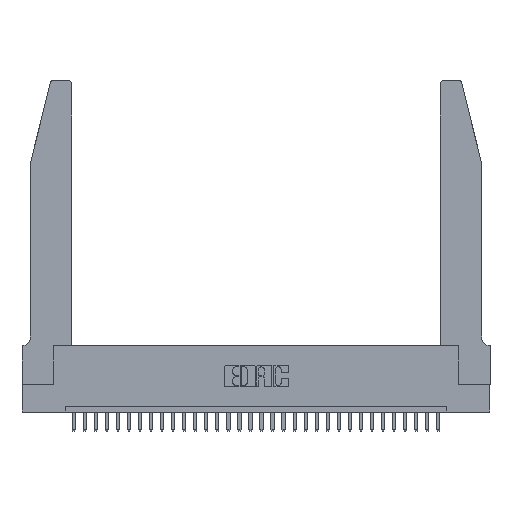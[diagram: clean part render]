
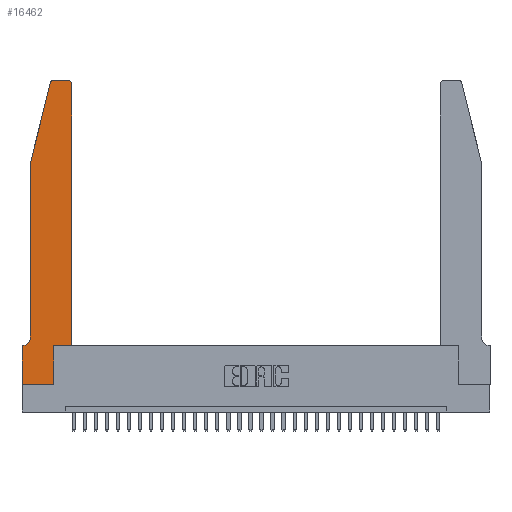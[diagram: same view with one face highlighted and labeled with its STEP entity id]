
A CAD part, top view. The second image highlights one B-rep face of the part: STEP entity #16462.
In plain terms, the highlighted planar face has unit normal (0, 0, 1).
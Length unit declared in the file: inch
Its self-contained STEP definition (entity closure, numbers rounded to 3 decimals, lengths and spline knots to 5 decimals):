
#124 = VECTOR ( 'NONE', #14231, 39.37008 ) ;
#172 = ORIENTED_EDGE ( 'NONE', *, *, #3746, .T. ) ;
#601 = VERTEX_POINT ( 'NONE', #12663 ) ;
#941 = VECTOR ( 'NONE', #10834, 39.37008 ) ;
#1388 = LINE ( 'NONE', #2856, #9377 ) ;
#1561 = VERTEX_POINT ( 'NONE', #30596 ) ;
#1982 = CARTESIAN_POINT ( 'NONE',  ( 0.2865, 0.35, 0.37 ) ) ;
#2059 = EDGE_CURVE ( 'NONE', #4789, #11589, #22545, .T. ) ;
#2856 = CARTESIAN_POINT ( 'NONE',  ( 0., 0., 0.37 ) ) ;
#2891 = AXIS2_PLACEMENT_3D ( 'NONE', #17776, #22571, #7738 ) ;
#2989 = CIRCLE ( 'NONE', #28407, 0.03 ) ;
#3746 = EDGE_CURVE ( 'NONE', #26715, #27314, #15465, .T. ) ;
#3977 = EDGE_CURVE ( 'NONE', #20438, #30515, #12324, .T. ) ;
#4060 = CARTESIAN_POINT ( 'NONE',  ( 0.0055, 0.42, 0.37 ) ) ;
#4115 = EDGE_LOOP ( 'NONE', ( #7812, #18271, #172, #4908, #11059, #21813, #10805, #12482, #27096, #6764, #14022, #16736 ) ) ;
#4284 = VECTOR ( 'NONE', #8783, 39.37008 ) ;
#4541 = CARTESIAN_POINT ( 'NONE',  ( 0.284, 2.72, 0.37 ) ) ;
#4668 = DIRECTION ( 'NONE',  ( 1., 0., 0. ) ) ;
#4789 = VERTEX_POINT ( 'NONE', #11998 ) ;
#4908 = ORIENTED_EDGE ( 'NONE', *, *, #10111, .T. ) ;
#5858 = CARTESIAN_POINT ( 'NONE',  ( 0.4205, 2.75, 0.37 ) ) ;
#6535 = LINE ( 'NONE', #1982, #124 ) ;
#6764 = ORIENTED_EDGE ( 'NONE', *, *, #2059, .T. ) ;
#7054 = AXIS2_PLACEMENT_3D ( 'NONE', #27290, #12754, #4668 ) ;
#7470 = LINE ( 'NONE', #10864, #19687 ) ;
#7738 = DIRECTION ( 'NONE',  ( 1., 0., 0. ) ) ;
#7812 = ORIENTED_EDGE ( 'NONE', *, *, #13483, .T. ) ;
#8783 = DIRECTION ( 'NONE',  ( 0., -1., 0. ) ) ;
#8975 = VECTOR ( 'NONE', #20133, 39.37008 ) ;
#9335 = EDGE_CURVE ( 'NONE', #16867, #601, #10926, .T. ) ;
#9377 = VECTOR ( 'NONE', #27277, 39.37008 ) ;
#10111 = EDGE_CURVE ( 'NONE', #27314, #16640, #26801, .T. ) ;
#10311 = EDGE_CURVE ( 'NONE', #30515, #4789, #6535, .T. ) ;
#10477 = CARTESIAN_POINT ( 'NONE',  ( 0.4505, 0.35, 0.37 ) ) ;
#10805 = ORIENTED_EDGE ( 'NONE', *, *, #28874, .T. ) ;
#10834 = DIRECTION ( 'NONE',  ( -0.239, -0.971, 0. ) ) ;
#10864 = CARTESIAN_POINT ( 'NONE',  ( 0.2605, 2.75, 0.37 ) ) ;
#10926 = LINE ( 'NONE', #27516, #8975 ) ;
#11059 = ORIENTED_EDGE ( 'NONE', *, *, #31287, .T. ) ;
#11589 = VERTEX_POINT ( 'NONE', #12778 ) ;
#11998 = CARTESIAN_POINT ( 'NONE',  ( 0.2865, 0.35, 0.37 ) ) ;
#12112 = EDGE_CURVE ( 'NONE', #1561, #15912, #23618, .T. ) ;
#12324 = LINE ( 'NONE', #30815, #23464 ) ;
#12482 = ORIENTED_EDGE ( 'NONE', *, *, #3977, .T. ) ;
#12663 = CARTESIAN_POINT ( 'NONE',  ( 0., 0.35, 0.37 ) ) ;
#12754 = DIRECTION ( 'NONE',  ( 0., 0., 1. ) ) ;
#12778 = CARTESIAN_POINT ( 'NONE',  ( 0.4505, 0.35, 0.37 ) ) ;
#12906 = CARTESIAN_POINT ( 'NONE',  ( 0., 0., 0.37 ) ) ;
#13483 = EDGE_CURVE ( 'NONE', #15912, #15859, #7470, .T. ) ;
#13767 = VECTOR ( 'NONE', #27560, 39.37008 ) ;
#13811 = VECTOR ( 'NONE', #16598, 39.37008 ) ;
#14022 = ORIENTED_EDGE ( 'NONE', *, *, #17224, .T. ) ;
#14231 = DIRECTION ( 'NONE',  ( 0., 1., 0. ) ) ;
#15142 = PLANE ( 'NONE',  #2891 ) ;
#15465 = LINE ( 'NONE', #25477, #941 ) ;
#15859 = VERTEX_POINT ( 'NONE', #27762 ) ;
#15912 = VERTEX_POINT ( 'NONE', #5858 ) ;
#16462 = ADVANCED_FACE ( 'NONE', ( #18083 ), #15142, .T. ) ;
#16598 = DIRECTION ( 'NONE',  ( 0., 1., 0. ) ) ;
#16640 = VERTEX_POINT ( 'NONE', #18291 ) ;
#16736 = ORIENTED_EDGE ( 'NONE', *, *, #12112, .T. ) ;
#16867 = VERTEX_POINT ( 'NONE', #21482 ) ;
#17224 = EDGE_CURVE ( 'NONE', #11589, #1561, #28723, .T. ) ;
#17776 = CARTESIAN_POINT ( 'NONE',  ( 0., 0.35, 0.37 ) ) ;
#18083 = FACE_OUTER_BOUND ( 'NONE', #4115, .T. ) ;
#18271 = ORIENTED_EDGE ( 'NONE', *, *, #27424, .T. ) ;
#18291 = CARTESIAN_POINT ( 'NONE',  ( 0.0755, 0.42, 0.37 ) ) ;
#19687 = VECTOR ( 'NONE', #28072, 39.37008 ) ;
#20133 = DIRECTION ( 'NONE',  ( -1., 0., 0. ) ) ;
#20438 = VERTEX_POINT ( 'NONE', #12906 ) ;
#20678 = DIRECTION ( 'NONE',  ( -1., 0., 0. ) ) ;
#20743 = CARTESIAN_POINT ( 'NONE',  ( 0.0755, 2., 0.37 ) ) ;
#21093 = DIRECTION ( 'NONE',  ( 0., 0., -1. ) ) ;
#21169 = CARTESIAN_POINT ( 'NONE',  ( 0.0755, 2., 0.37 ) ) ;
#21482 = CARTESIAN_POINT ( 'NONE',  ( 0.0055, 0.35, 0.37 ) ) ;
#21588 = DIRECTION ( 'NONE',  ( 0., 0., 1. ) ) ;
#21598 = CARTESIAN_POINT ( 'NONE',  ( 0.4505, 0.35, 0.37 ) ) ;
#21813 = ORIENTED_EDGE ( 'NONE', *, *, #9335, .T. ) ;
#22545 = LINE ( 'NONE', #10477, #13767 ) ;
#22558 = CIRCLE ( 'NONE', #25610, 0.07 ) ;
#22571 = DIRECTION ( 'NONE',  ( 0., 0., 1. ) ) ;
#23448 = CARTESIAN_POINT ( 'NONE',  ( 0.25487, 2.72718, 0.37 ) ) ;
#23464 = VECTOR ( 'NONE', #30249, 39.37008 ) ;
#23618 = CIRCLE ( 'NONE', #7054, 0.03 ) ;
#25477 = CARTESIAN_POINT ( 'NONE',  ( 0.0755, 2., 0.37 ) ) ;
#25610 = AXIS2_PLACEMENT_3D ( 'NONE', #4060, #21093, #20678 ) ;
#26553 = CARTESIAN_POINT ( 'NONE',  ( 0.2865, 0., 0.37 ) ) ;
#26715 = VERTEX_POINT ( 'NONE', #23448 ) ;
#26801 = LINE ( 'NONE', #20743, #4284 ) ;
#27096 = ORIENTED_EDGE ( 'NONE', *, *, #10311, .T. ) ;
#27277 = DIRECTION ( 'NONE',  ( 0., -1., 0. ) ) ;
#27290 = CARTESIAN_POINT ( 'NONE',  ( 0.4205, 2.72, 0.37 ) ) ;
#27314 = VERTEX_POINT ( 'NONE', #21169 ) ;
#27424 = EDGE_CURVE ( 'NONE', #15859, #26715, #2989, .T. ) ;
#27516 = CARTESIAN_POINT ( 'NONE',  ( 0.0755, 0.35, 0.37 ) ) ;
#27560 = DIRECTION ( 'NONE',  ( 1., 0., 0. ) ) ;
#27762 = CARTESIAN_POINT ( 'NONE',  ( 0.284, 2.75, 0.37 ) ) ;
#28072 = DIRECTION ( 'NONE',  ( -1., 0., 0. ) ) ;
#28407 = AXIS2_PLACEMENT_3D ( 'NONE', #4541, #21588, #31409 ) ;
#28723 = LINE ( 'NONE', #21598, #13811 ) ;
#28874 = EDGE_CURVE ( 'NONE', #601, #20438, #1388, .T. ) ;
#30249 = DIRECTION ( 'NONE',  ( 1., 0., 0. ) ) ;
#30515 = VERTEX_POINT ( 'NONE', #26553 ) ;
#30596 = CARTESIAN_POINT ( 'NONE',  ( 0.4505, 2.72, 0.37 ) ) ;
#30815 = CARTESIAN_POINT ( 'NONE',  ( 0., 0., 0.37 ) ) ;
#31287 = EDGE_CURVE ( 'NONE', #16640, #16867, #22558, .T. ) ;
#31409 = DIRECTION ( 'NONE',  ( 1., 0., 0. ) ) ;
